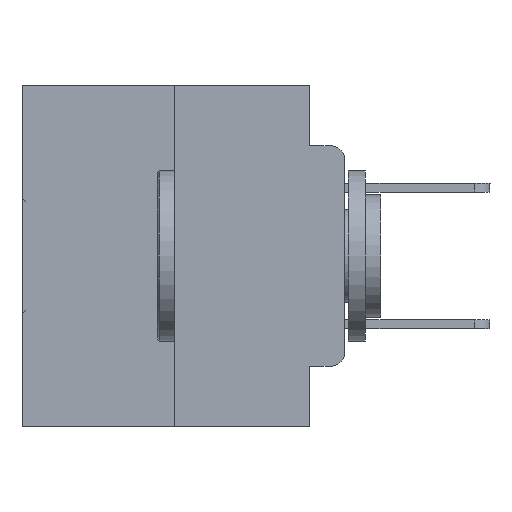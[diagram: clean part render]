
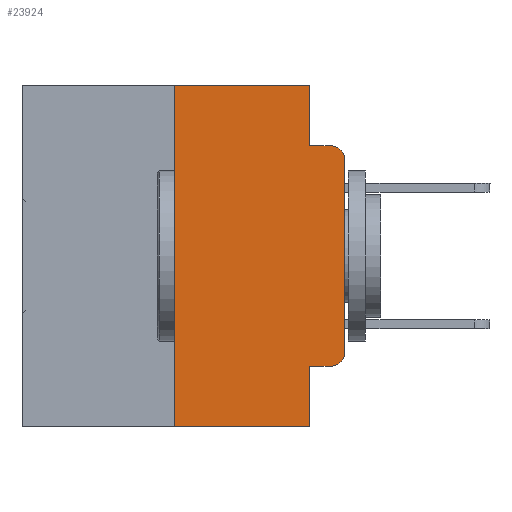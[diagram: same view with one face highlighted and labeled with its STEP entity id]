
A CAD part, left-side view. The second image highlights one B-rep face of the part: STEP entity #23924.
In plain terms, the highlighted planar face has unit normal (-1, 0, 0).
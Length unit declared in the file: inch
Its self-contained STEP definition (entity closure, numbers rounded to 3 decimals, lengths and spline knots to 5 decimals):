
#221 = ORIENTED_EDGE ( 'NONE', *, *, #25865, .F. ) ;
#597 = DIRECTION ( 'NONE',  ( -1., 0., 0. ) ) ;
#903 = VERTEX_POINT ( 'NONE', #11605 ) ;
#1201 = PLANE ( 'NONE',  #28533 ) ;
#1573 = AXIS2_PLACEMENT_3D ( 'NONE', #15605, #597, #18065 ) ;
#2015 = VERTEX_POINT ( 'NONE', #15744 ) ;
#3019 = VERTEX_POINT ( 'NONE', #7434 ) ;
#3112 = DIRECTION ( 'NONE',  ( 0., 0., -1. ) ) ;
#3771 = DIRECTION ( 'NONE',  ( 1., 0., 0. ) ) ;
#3818 = EDGE_CURVE ( 'NONE', #19038, #13552, #15132, .T. ) ;
#4105 = EDGE_CURVE ( 'NONE', #15293, #903, #12458, .T. ) ;
#4188 = VECTOR ( 'NONE', #23579, 39.37008 ) ;
#4262 = EDGE_CURVE ( 'NONE', #24752, #3019, #15099, .T. ) ;
#4445 = DIRECTION ( 'NONE',  ( 0., 0., 1. ) ) ;
#5546 = EDGE_CURVE ( 'NONE', #2015, #13552, #30147, .T. ) ;
#5562 = CARTESIAN_POINT ( 'NONE',  ( 0., 0.02, -0.0885 ) ) ;
#5848 = VECTOR ( 'NONE', #23973, 39.37008 ) ;
#5891 = CARTESIAN_POINT ( 'NONE',  ( 0., 0.02, -0.3915 ) ) ;
#6368 = CIRCLE ( 'NONE', #22868, 0.02 ) ;
#7297 = EDGE_CURVE ( 'NONE', #9433, #2015, #30852, .T. ) ;
#7434 = CARTESIAN_POINT ( 'NONE',  ( 0., 0.051, -0.5 ) ) ;
#7714 = DIRECTION ( 'NONE',  ( 0., 0., 1. ) ) ;
#8482 = DIRECTION ( 'NONE',  ( 0., 0., -1. ) ) ;
#9433 = VERTEX_POINT ( 'NONE', #21398 ) ;
#10216 = ORIENTED_EDGE ( 'NONE', *, *, #17755, .T. ) ;
#10606 = LINE ( 'NONE', #22269, #29156 ) ;
#10788 = VECTOR ( 'NONE', #4445, 39.37008 ) ;
#11311 = ORIENTED_EDGE ( 'NONE', *, *, #27442, .F. ) ;
#11410 = CARTESIAN_POINT ( 'NONE',  ( 0., 0.02, -0.4115 ) ) ;
#11605 = CARTESIAN_POINT ( 'NONE',  ( 0., 0.051, 0. ) ) ;
#12458 = LINE ( 'NONE', #16388, #5848 ) ;
#12838 = ORIENTED_EDGE ( 'NONE', *, *, #4105, .F. ) ;
#13552 = VERTEX_POINT ( 'NONE', #5562 ) ;
#14349 = FACE_OUTER_BOUND ( 'NONE', #20449, .T. ) ;
#14381 = VECTOR ( 'NONE', #30089, 39.37008 ) ;
#14746 = DIRECTION ( 'NONE',  ( 0., -1., 0. ) ) ;
#14772 = CARTESIAN_POINT ( 'NONE',  ( 0., 0.25, 0. ) ) ;
#15099 = LINE ( 'NONE', #26844, #20858 ) ;
#15125 = ORIENTED_EDGE ( 'NONE', *, *, #21025, .F. ) ;
#15132 = LINE ( 'NONE', #15630, #14381 ) ;
#15293 = VERTEX_POINT ( 'NONE', #14772 ) ;
#15605 = CARTESIAN_POINT ( 'NONE',  ( 0., 0.02, -0.1085 ) ) ;
#15630 = CARTESIAN_POINT ( 'NONE',  ( 0., 0.051, -0.0885 ) ) ;
#15744 = CARTESIAN_POINT ( 'NONE',  ( 0., 0., -0.1085 ) ) ;
#16388 = CARTESIAN_POINT ( 'NONE',  ( 0., 0.473, 0. ) ) ;
#17292 = LINE ( 'NONE', #21729, #10788 ) ;
#17755 = EDGE_CURVE ( 'NONE', #21791, #9433, #6368, .T. ) ;
#18065 = DIRECTION ( 'NONE',  ( 0., 0., -1. ) ) ;
#18636 = CARTESIAN_POINT ( 'NONE',  ( 0., 0.473, 0. ) ) ;
#19038 = VERTEX_POINT ( 'NONE', #25834 ) ;
#19400 = EDGE_CURVE ( 'NONE', #23009, #21791, #10606, .T. ) ;
#20029 = LINE ( 'NONE', #20420, #25704 ) ;
#20420 = CARTESIAN_POINT ( 'NONE',  ( 0., 0.051, 0. ) ) ;
#20449 = EDGE_LOOP ( 'NONE', ( #20479, #21246, #23559, #11311, #12838, #221, #27253, #15125, #27989, #10216 ) ) ;
#20479 = ORIENTED_EDGE ( 'NONE', *, *, #7297, .T. ) ;
#20858 = VECTOR ( 'NONE', #14746, 39.37008 ) ;
#21025 = EDGE_CURVE ( 'NONE', #23009, #3019, #20029, .T. ) ;
#21087 = DIRECTION ( 'NONE',  ( 0., 0., -1. ) ) ;
#21246 = ORIENTED_EDGE ( 'NONE', *, *, #5546, .T. ) ;
#21398 = CARTESIAN_POINT ( 'NONE',  ( 0., 0., -0.3915 ) ) ;
#21729 = CARTESIAN_POINT ( 'NONE',  ( 0., 0.25, 0. ) ) ;
#21791 = VERTEX_POINT ( 'NONE', #11410 ) ;
#22269 = CARTESIAN_POINT ( 'NONE',  ( 0., 0.051, -0.4115 ) ) ;
#22868 = AXIS2_PLACEMENT_3D ( 'NONE', #5891, #23114, #8482 ) ;
#23009 = VERTEX_POINT ( 'NONE', #26706 ) ;
#23114 = DIRECTION ( 'NONE',  ( -1., 0., 0. ) ) ;
#23559 = ORIENTED_EDGE ( 'NONE', *, *, #3818, .F. ) ;
#23579 = DIRECTION ( 'NONE',  ( 0., 0., -1. ) ) ;
#23924 = ADVANCED_FACE ( 'NONE', ( #14349 ), #1201, .F. ) ;
#23973 = DIRECTION ( 'NONE',  ( 0., -1., 0. ) ) ;
#24147 = CARTESIAN_POINT ( 'NONE',  ( 0., 0.25, -0.5 ) ) ;
#24752 = VERTEX_POINT ( 'NONE', #24147 ) ;
#24801 = DIRECTION ( 'NONE',  ( 0., -1., 0. ) ) ;
#25704 = VECTOR ( 'NONE', #3112, 39.37008 ) ;
#25834 = CARTESIAN_POINT ( 'NONE',  ( 0., 0.051, -0.0885 ) ) ;
#25865 = EDGE_CURVE ( 'NONE', #24752, #15293, #17292, .T. ) ;
#26706 = CARTESIAN_POINT ( 'NONE',  ( 0., 0.051, -0.4115 ) ) ;
#26844 = CARTESIAN_POINT ( 'NONE',  ( 0., 0.473, -0.5 ) ) ;
#27253 = ORIENTED_EDGE ( 'NONE', *, *, #4262, .T. ) ;
#27442 = EDGE_CURVE ( 'NONE', #903, #19038, #29448, .T. ) ;
#27989 = ORIENTED_EDGE ( 'NONE', *, *, #19400, .T. ) ;
#28314 = CARTESIAN_POINT ( 'NONE',  ( 0., 0.051, 0. ) ) ;
#28533 = AXIS2_PLACEMENT_3D ( 'NONE', #18636, #3771, #21087 ) ;
#29156 = VECTOR ( 'NONE', #24801, 39.37008 ) ;
#29448 = LINE ( 'NONE', #28314, #4188 ) ;
#29548 = CARTESIAN_POINT ( 'NONE',  ( 0., 0., 0. ) ) ;
#30089 = DIRECTION ( 'NONE',  ( 0., -1., 0. ) ) ;
#30094 = VECTOR ( 'NONE', #7714, 39.37008 ) ;
#30147 = CIRCLE ( 'NONE', #1573, 0.02 ) ;
#30852 = LINE ( 'NONE', #29548, #30094 ) ;
